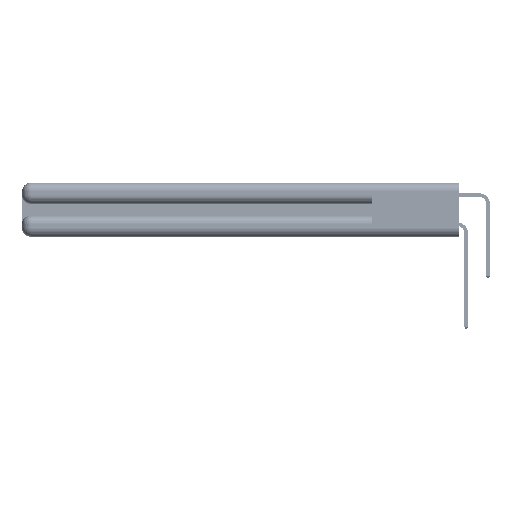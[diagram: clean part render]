
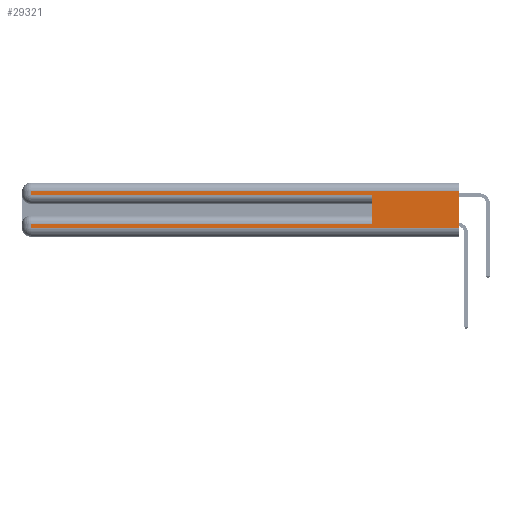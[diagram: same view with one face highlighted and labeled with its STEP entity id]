
A CAD part, left-side view. The second image highlights one B-rep face of the part: STEP entity #29321.
In plain terms, the highlighted planar face has unit normal (-1, 0, 0).
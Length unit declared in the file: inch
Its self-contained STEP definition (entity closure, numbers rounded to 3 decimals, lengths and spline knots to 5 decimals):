
#2298 = CARTESIAN_POINT ( 'NONE',  ( 0., 2.94, 0.085 ) ) ;
#3556 = LINE ( 'NONE', #5034, #45523 ) ;
#5034 = CARTESIAN_POINT ( 'NONE',  ( 0., 0.6, 0.145 ) ) ;
#5498 = VECTOR ( 'NONE', #21085, 39.37008 ) ;
#6273 = AXIS2_PLACEMENT_3D ( 'NONE', #12714, #17083, #47347 ) ;
#8008 = CARTESIAN_POINT ( 'NONE',  ( 0., 2.94, 0.37 ) ) ;
#10215 = EDGE_CURVE ( 'NONE', #46316, #26325, #47356, .T. ) ;
#10241 = ORIENTED_EDGE ( 'NONE', *, *, #32139, .T. ) ;
#10944 = DIRECTION ( 'NONE',  ( 0., -1., 0. ) ) ;
#12714 = CARTESIAN_POINT ( 'NONE',  ( 0., 0., 0.37 ) ) ;
#12777 = VERTEX_POINT ( 'NONE', #27038 ) ;
#12804 = VECTOR ( 'NONE', #24327, 39.37008 ) ;
#14203 = EDGE_CURVE ( 'NONE', #24997, #55357, #55053, .T. ) ;
#16910 = ORIENTED_EDGE ( 'NONE', *, *, #24495, .F. ) ;
#17013 = LINE ( 'NONE', #8008, #5498 ) ;
#17083 = DIRECTION ( 'NONE',  ( 1., 0., 0. ) ) ;
#17250 = VERTEX_POINT ( 'NONE', #40574 ) ;
#17266 = CARTESIAN_POINT ( 'NONE',  ( 0., 2.94, 0.285 ) ) ;
#18086 = DIRECTION ( 'NONE',  ( 0., 0., -1. ) ) ;
#20527 = EDGE_CURVE ( 'NONE', #26325, #22073, #34419, .T. ) ;
#21085 = DIRECTION ( 'NONE',  ( 0., 0., -1. ) ) ;
#22073 = VERTEX_POINT ( 'NONE', #34791 ) ;
#22958 = VECTOR ( 'NONE', #41163, 39.37008 ) ;
#24052 = CARTESIAN_POINT ( 'NONE',  ( 0., 0., 0.285 ) ) ;
#24327 = DIRECTION ( 'NONE',  ( 0., 1., 0. ) ) ;
#24495 = EDGE_CURVE ( 'NONE', #46316, #55357, #3556, .T. ) ;
#24997 = VERTEX_POINT ( 'NONE', #17266 ) ;
#25132 = LINE ( 'NONE', #45586, #46775 ) ;
#25435 = EDGE_CURVE ( 'NONE', #22073, #47546, #25132, .T. ) ;
#26325 = VERTEX_POINT ( 'NONE', #2298 ) ;
#26790 = DIRECTION ( 'NONE',  ( 0., 0., 1. ) ) ;
#27038 = CARTESIAN_POINT ( 'NONE',  ( 0., 2.94, 0.31 ) ) ;
#29321 = ADVANCED_FACE ( 'NONE', ( #40891 ), #38618, .F. ) ;
#29555 = CARTESIAN_POINT ( 'NONE',  ( 0., 0.6, 0.085 ) ) ;
#30591 = ORIENTED_EDGE ( 'NONE', *, *, #14203, .T. ) ;
#31116 = CARTESIAN_POINT ( 'NONE',  ( 0., 0., 0.37 ) ) ;
#31398 = CARTESIAN_POINT ( 'NONE',  ( 0., 0.6, 0.285 ) ) ;
#31555 = CARTESIAN_POINT ( 'NONE',  ( 0., 0., 0.06 ) ) ;
#31582 = EDGE_CURVE ( 'NONE', #12777, #24997, #17013, .T. ) ;
#32139 = EDGE_CURVE ( 'NONE', #17250, #12777, #44709, .T. ) ;
#33327 = CARTESIAN_POINT ( 'NONE',  ( 0., 0., 0.31 ) ) ;
#34291 = ORIENTED_EDGE ( 'NONE', *, *, #34730, .F. ) ;
#34419 = LINE ( 'NONE', #54058, #22958 ) ;
#34730 = EDGE_CURVE ( 'NONE', #17250, #47546, #37213, .T. ) ;
#34791 = CARTESIAN_POINT ( 'NONE',  ( 0., 2.94, 0.06 ) ) ;
#36277 = ORIENTED_EDGE ( 'NONE', *, *, #20527, .T. ) ;
#37213 = LINE ( 'NONE', #31116, #48740 ) ;
#37659 = DIRECTION ( 'NONE',  ( 0., 1., 0. ) ) ;
#38430 = ORIENTED_EDGE ( 'NONE', *, *, #25435, .T. ) ;
#38618 = PLANE ( 'NONE',  #6273 ) ;
#40574 = CARTESIAN_POINT ( 'NONE',  ( 0., 0., 0.31 ) ) ;
#40891 = FACE_OUTER_BOUND ( 'NONE', #51172, .T. ) ;
#41163 = DIRECTION ( 'NONE',  ( 0., 0., -1. ) ) ;
#43538 = VECTOR ( 'NONE', #10944, 39.37008 ) ;
#44709 = LINE ( 'NONE', #33327, #53526 ) ;
#44864 = ORIENTED_EDGE ( 'NONE', *, *, #31582, .T. ) ;
#45523 = VECTOR ( 'NONE', #26790, 39.37008 ) ;
#45586 = CARTESIAN_POINT ( 'NONE',  ( 0., 0., 0.06 ) ) ;
#45872 = CARTESIAN_POINT ( 'NONE',  ( 0., 0., 0.085 ) ) ;
#46316 = VERTEX_POINT ( 'NONE', #29555 ) ;
#46775 = VECTOR ( 'NONE', #49947, 39.37008 ) ;
#47347 = DIRECTION ( 'NONE',  ( 0., 0., -1. ) ) ;
#47356 = LINE ( 'NONE', #45872, #12804 ) ;
#47546 = VERTEX_POINT ( 'NONE', #31555 ) ;
#48740 = VECTOR ( 'NONE', #18086, 39.37008 ) ;
#49947 = DIRECTION ( 'NONE',  ( 0., -1., 0. ) ) ;
#51172 = EDGE_LOOP ( 'NONE', ( #34291, #10241, #44864, #30591, #16910, #52871, #36277, #38430 ) ) ;
#52871 = ORIENTED_EDGE ( 'NONE', *, *, #10215, .T. ) ;
#53526 = VECTOR ( 'NONE', #37659, 39.37008 ) ;
#54058 = CARTESIAN_POINT ( 'NONE',  ( 0., 2.94, 0.37 ) ) ;
#55053 = LINE ( 'NONE', #24052, #43538 ) ;
#55357 = VERTEX_POINT ( 'NONE', #31398 ) ;
